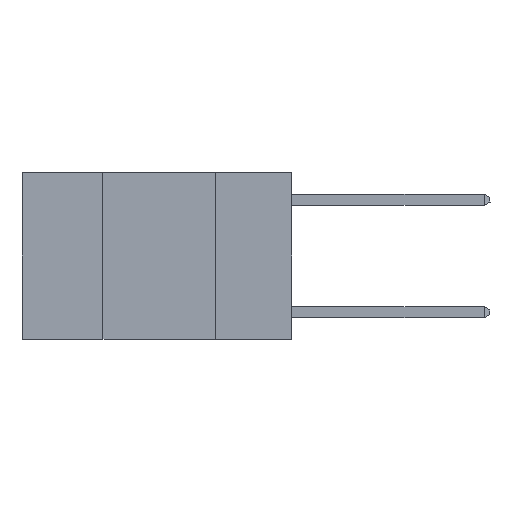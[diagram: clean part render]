
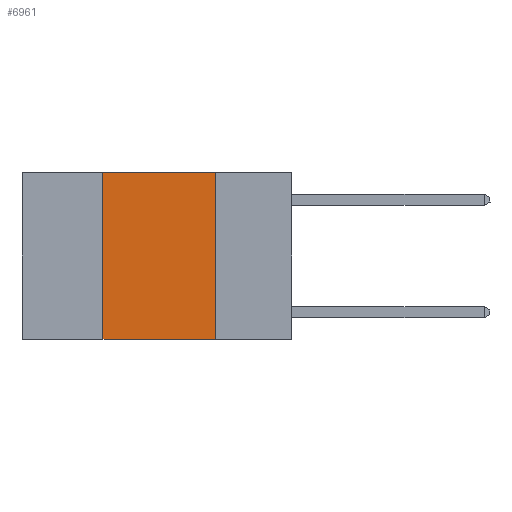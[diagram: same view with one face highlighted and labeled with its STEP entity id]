
A CAD part, left-side view. The second image highlights one B-rep face of the part: STEP entity #6961.
In plain terms, the highlighted planar face has unit normal (-1, 0, 0).
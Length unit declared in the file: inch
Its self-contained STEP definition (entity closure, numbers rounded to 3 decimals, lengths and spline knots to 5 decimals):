
#2343 = EDGE_CURVE ( 'NONE', #5818, #11443, #13268, .T. ) ;
#2591 = PLANE ( 'NONE',  #13426 ) ;
#2943 = LINE ( 'NONE', #4382, #12427 ) ;
#3695 = LINE ( 'NONE', #9751, #13170 ) ;
#3840 = EDGE_CURVE ( 'NONE', #11364, #5818, #2943, .T. ) ;
#3907 = DIRECTION ( 'NONE',  ( 0., 0., -1. ) ) ;
#4382 = CARTESIAN_POINT ( 'NONE',  ( 0., 0.42, 0. ) ) ;
#4782 = CARTESIAN_POINT ( 'NONE',  ( 0., 0.42, -0.37 ) ) ;
#5818 = VERTEX_POINT ( 'NONE', #14156 ) ;
#6334 = EDGE_CURVE ( 'NONE', #11364, #14109, #15438, .T. ) ;
#6961 = ADVANCED_FACE ( 'NONE', ( #7289 ), #2591, .F. ) ;
#7289 = FACE_OUTER_BOUND ( 'NONE', #10982, .T. ) ;
#7706 = CARTESIAN_POINT ( 'NONE',  ( 0., 0.6, -0.37 ) ) ;
#8546 = ORIENTED_EDGE ( 'NONE', *, *, #13210, .F. ) ;
#8772 = CARTESIAN_POINT ( 'NONE',  ( 0., 0.17, 0. ) ) ;
#8805 = ORIENTED_EDGE ( 'NONE', *, *, #2343, .F. ) ;
#9719 = ORIENTED_EDGE ( 'NONE', *, *, #3840, .F. ) ;
#9751 = CARTESIAN_POINT ( 'NONE',  ( 0., 0.17, 0. ) ) ;
#10011 = CARTESIAN_POINT ( 'NONE',  ( 0., 0.6, 0. ) ) ;
#10339 = ORIENTED_EDGE ( 'NONE', *, *, #6334, .T. ) ;
#10850 = VECTOR ( 'NONE', #12770, 39.37008 ) ;
#10982 = EDGE_LOOP ( 'NONE', ( #8546, #8805, #9719, #10339 ) ) ;
#11011 = DIRECTION ( 'NONE',  ( 0., 0., -1. ) ) ;
#11257 = DIRECTION ( 'NONE',  ( 1., 0., 0. ) ) ;
#11364 = VERTEX_POINT ( 'NONE', #4782 ) ;
#11443 = VERTEX_POINT ( 'NONE', #8772 ) ;
#11481 = CARTESIAN_POINT ( 'NONE',  ( 0., 0.6, 0. ) ) ;
#11709 = DIRECTION ( 'NONE',  ( 0., 0., 1. ) ) ;
#12080 = VECTOR ( 'NONE', #13866, 39.37008 ) ;
#12427 = VECTOR ( 'NONE', #11709, 39.37008 ) ;
#12770 = DIRECTION ( 'NONE',  ( 0., -1., 0. ) ) ;
#13170 = VECTOR ( 'NONE', #11011, 39.37008 ) ;
#13210 = EDGE_CURVE ( 'NONE', #11443, #14109, #3695, .T. ) ;
#13268 = LINE ( 'NONE', #11481, #10850 ) ;
#13426 = AXIS2_PLACEMENT_3D ( 'NONE', #10011, #11257, #3907 ) ;
#13866 = DIRECTION ( 'NONE',  ( 0., -1., 0. ) ) ;
#14109 = VERTEX_POINT ( 'NONE', #15077 ) ;
#14156 = CARTESIAN_POINT ( 'NONE',  ( 0., 0.42, 0. ) ) ;
#15077 = CARTESIAN_POINT ( 'NONE',  ( 0., 0.17, -0.37 ) ) ;
#15438 = LINE ( 'NONE', #7706, #12080 ) ;
